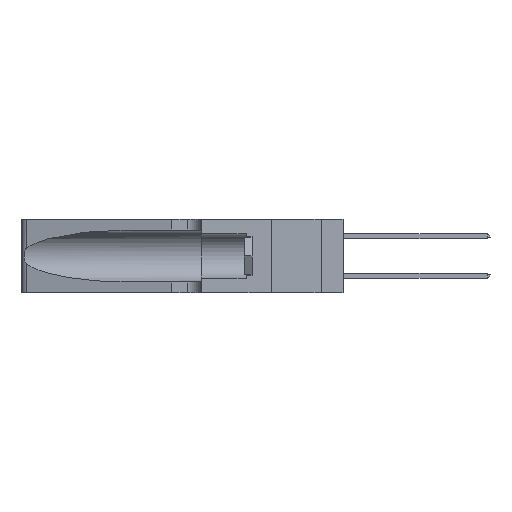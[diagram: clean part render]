
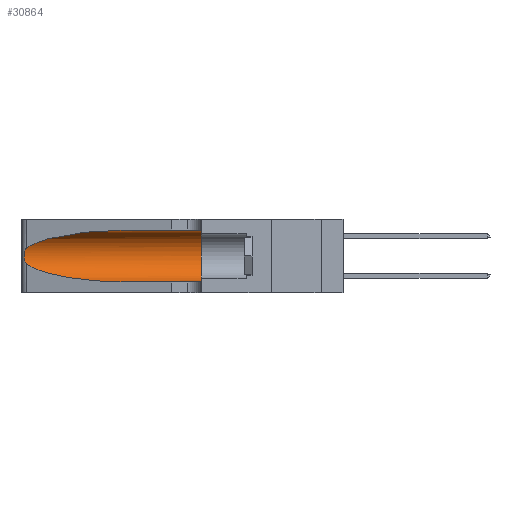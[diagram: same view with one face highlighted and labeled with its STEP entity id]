
A CAD part, left-side view. The second image highlights one B-rep face of the part: STEP entity #30864.
In plain terms, the highlighted cylindrical face has radius 3.308 mm (diameter 6.617 mm), a partial arc.
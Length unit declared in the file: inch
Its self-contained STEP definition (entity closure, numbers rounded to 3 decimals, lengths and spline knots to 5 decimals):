
#202 = CARTESIAN_POINT ( 'NONE',  ( 0.1305, 1.61858, 0.185 ) ) ;
#252 = VECTOR ( 'NONE', #2765, 39.37008 ) ;
#1918 = VERTEX_POINT ( 'NONE', #35611 ) ;
#2190 = EDGE_CURVE ( 'NONE', #16565, #1918, #16010, .T. ) ;
#2278 = EDGE_CURVE ( 'NONE', #1918, #22411, #9287, .T. ) ;
#2765 = DIRECTION ( 'NONE',  ( 0., -1., 0. ) ) ;
#3596 = ORIENTED_EDGE ( 'NONE', *, *, #27145, .F. ) ;
#3801 = EDGE_CURVE ( 'NONE', #22411, #33654, #17924, .T. ) ;
#4115 = CARTESIAN_POINT ( 'NONE',  ( 0.25639, 1.23184, 0.21858 ) ) ;
#4434 = VERTEX_POINT ( 'NONE', #35431 ) ;
#4973 = CARTESIAN_POINT ( 'NONE',  ( 0.25856, 1.23593, 0.16098 ) ) ;
#5392 = CARTESIAN_POINT ( 'NONE',  ( 0.25639, 1.23186, 0.15144 ) ) ;
#5535 = AXIS2_PLACEMENT_3D ( 'NONE', #42861, #26240, #29584 ) ;
#7870 = CARTESIAN_POINT ( 'NONE',  ( 0.26018, 1.23835, 0.19895 ) ) ;
#8505 = VERTEX_POINT ( 'NONE', #13565 ) ;
#9287 =( BOUNDED_CURVE ( )  B_SPLINE_CURVE ( 3, ( #32951, #29862, #23445, #36570 ),
 .UNSPECIFIED., .F., .F. ) 
 B_SPLINE_CURVE_WITH_KNOTS ( ( 4, 4 ),
 ( 3.44316, 4.71239 ),
 .UNSPECIFIED. ) 
 CURVE ( )  GEOMETRIC_REPRESENTATION_ITEM ( )  RATIONAL_B_SPLINE_CURVE ( ( 1., 0.87, 0.87, 1. ) ) 
 REPRESENTATION_ITEM ( '' )  );
#10421 = DIRECTION ( 'NONE',  ( 0., 0., -1. ) ) ;
#11512 = CARTESIAN_POINT ( 'NONE',  ( 0.25487, 1.22718, 0.22369 ) ) ;
#13412 = FACE_OUTER_BOUND ( 'NONE', #41777, .T. ) ;
#13565 = CARTESIAN_POINT ( 'NONE',  ( 0.1305, 0.72297, 0.31525 ) ) ;
#14014 = CARTESIAN_POINT ( 'NONE',  ( 0.1305, 1.61858, 0.31525 ) ) ;
#15366 = ORIENTED_EDGE ( 'NONE', *, *, #2278, .T. ) ;
#16010 = B_SPLINE_CURVE_WITH_KNOTS ( 'NONE', 3,
 ( #36373, #23107, #4115, #34288, #34877, #7870, #34442, #28037, #31405, #4973, #41853, #5392, #21909, #31982 ),
 .UNSPECIFIED., .F., .F.,
 ( 4, 2, 2, 2, 2, 2, 4 ),
 ( 0., 0.00027, 0.00053, 0.00107, 0.0016, 0.00187, 0.00214 ),
 .UNSPECIFIED. ) ;
#16105 = CARTESIAN_POINT ( 'NONE',  ( 0.1305, 1.61858, 0.05475 ) ) ;
#16433 = AXIS2_PLACEMENT_3D ( 'NONE', #202, #29688, #10421 ) ;
#16565 = VERTEX_POINT ( 'NONE', #27830 ) ;
#17924 = LINE ( 'NONE', #16105, #252 ) ;
#18697 = VECTOR ( 'NONE', #26943, 39.37008 ) ;
#20802 = ORIENTED_EDGE ( 'NONE', *, *, #2190, .T. ) ;
#21369 = CARTESIAN_POINT ( 'NONE',  ( 0.2373, 1.15595, 0.28018 ) ) ;
#21909 = CARTESIAN_POINT ( 'NONE',  ( 0.25555, 1.22993, 0.14849 ) ) ;
#22031 =( BOUNDED_CURVE ( )  B_SPLINE_CURVE ( 3, ( #30973, #24413, #21369, #11512 ),
 .UNSPECIFIED., .F., .F. ) 
 B_SPLINE_CURVE_WITH_KNOTS ( ( 4, 4 ),
 ( 1.5708, 2.84003 ),
 .UNSPECIFIED. ) 
 CURVE ( )  GEOMETRIC_REPRESENTATION_ITEM ( )  RATIONAL_B_SPLINE_CURVE ( ( 1., 0.87, 0.87, 1. ) ) 
 REPRESENTATION_ITEM ( '' )  );
#22411 = VERTEX_POINT ( 'NONE', #29120 ) ;
#23107 = CARTESIAN_POINT ( 'NONE',  ( 0.25555, 1.22994, 0.2215 ) ) ;
#23445 = CARTESIAN_POINT ( 'NONE',  ( 0.18966, 0.96281, 0.05475 ) ) ;
#24337 = CYLINDRICAL_SURFACE ( 'NONE', #16433, 0.13025 ) ;
#24413 = CARTESIAN_POINT ( 'NONE',  ( 0.18966, 0.96281, 0.31525 ) ) ;
#26240 = DIRECTION ( 'NONE',  ( 0., 1., 0. ) ) ;
#26943 = DIRECTION ( 'NONE',  ( 0., -1., 0. ) ) ;
#27145 = EDGE_CURVE ( 'NONE', #4434, #33654, #31404, .T. ) ;
#27217 = ORIENTED_EDGE ( 'NONE', *, *, #3801, .T. ) ;
#27830 = CARTESIAN_POINT ( 'NONE',  ( 0.25487, 1.22718, 0.22369 ) ) ;
#28037 = CARTESIAN_POINT ( 'NONE',  ( 0.26075, 1.23896, 0.178 ) ) ;
#29109 = CARTESIAN_POINT ( 'NONE',  ( 0.1305, 0.35, 0.05475 ) ) ;
#29120 = CARTESIAN_POINT ( 'NONE',  ( 0.1305, 0.72297, 0.05475 ) ) ;
#29584 = DIRECTION ( 'NONE',  ( 0., 0., 1. ) ) ;
#29688 = DIRECTION ( 'NONE',  ( 0., -1., 0. ) ) ;
#29862 = CARTESIAN_POINT ( 'NONE',  ( 0.2373, 1.15595, 0.08982 ) ) ;
#30864 = ADVANCED_FACE ( 'NONE', ( #13412 ), #24337, .F. ) ;
#30973 = CARTESIAN_POINT ( 'NONE',  ( 0.1305, 0.72297, 0.31525 ) ) ;
#31404 = CIRCLE ( 'NONE', #5535, 0.13025 ) ;
#31405 = CARTESIAN_POINT ( 'NONE',  ( 0.26017, 1.23833, 0.17102 ) ) ;
#31982 = CARTESIAN_POINT ( 'NONE',  ( 0.25487, 1.22718, 0.14631 ) ) ;
#32804 = ORIENTED_EDGE ( 'NONE', *, *, #41315, .T. ) ;
#32951 = CARTESIAN_POINT ( 'NONE',  ( 0.25487, 1.22718, 0.14631 ) ) ;
#33149 = EDGE_CURVE ( 'NONE', #8505, #4434, #38483, .T. ) ;
#33654 = VERTEX_POINT ( 'NONE', #29109 ) ;
#34288 = CARTESIAN_POINT ( 'NONE',  ( 0.25787, 1.23484, 0.2124 ) ) ;
#34442 = CARTESIAN_POINT ( 'NONE',  ( 0.26075, 1.23896, 0.19203 ) ) ;
#34877 = CARTESIAN_POINT ( 'NONE',  ( 0.25854, 1.2359, 0.20912 ) ) ;
#35431 = CARTESIAN_POINT ( 'NONE',  ( 0.1305, 0.35, 0.31525 ) ) ;
#35611 = CARTESIAN_POINT ( 'NONE',  ( 0.25487, 1.22718, 0.14631 ) ) ;
#36373 = CARTESIAN_POINT ( 'NONE',  ( 0.25487, 1.22718, 0.22369 ) ) ;
#36570 = CARTESIAN_POINT ( 'NONE',  ( 0.1305, 0.72297, 0.05475 ) ) ;
#38483 = LINE ( 'NONE', #14014, #18697 ) ;
#39712 = ORIENTED_EDGE ( 'NONE', *, *, #33149, .F. ) ;
#41315 = EDGE_CURVE ( 'NONE', #8505, #16565, #22031, .T. ) ;
#41777 = EDGE_LOOP ( 'NONE', ( #32804, #20802, #15366, #27217, #3596, #39712 ) ) ;
#41853 = CARTESIAN_POINT ( 'NONE',  ( 0.25789, 1.23486, 0.15765 ) ) ;
#42861 = CARTESIAN_POINT ( 'NONE',  ( 0.1305, 0.35, 0.185 ) ) ;
